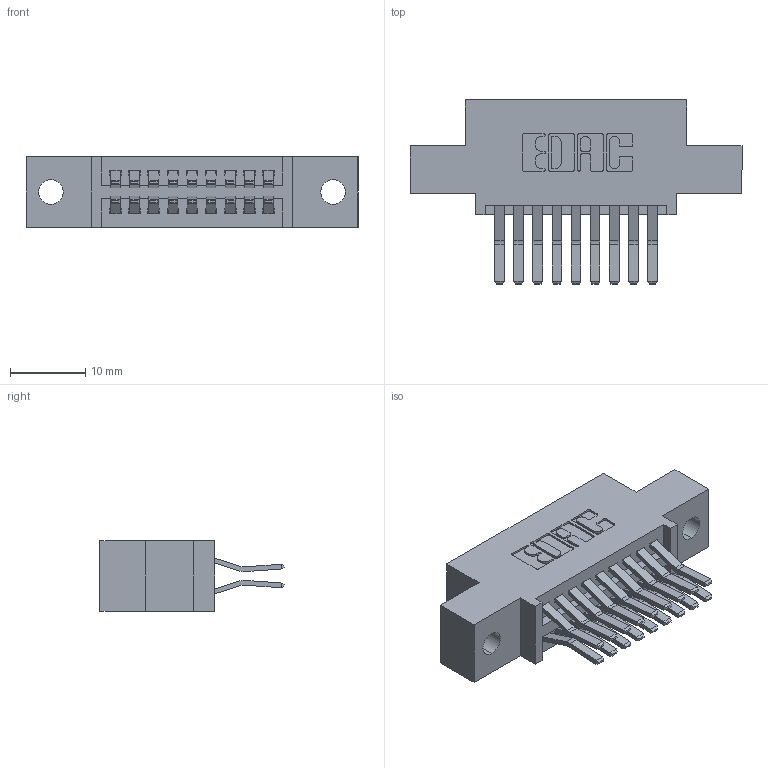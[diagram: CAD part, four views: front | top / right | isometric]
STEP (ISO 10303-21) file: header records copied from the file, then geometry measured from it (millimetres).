
FILE_DESCRIPTION (( 'STEP AP203' ), '1' );
FILE_NAME ('345-018-560-502.STEP', '2019-10-27T07:20:52', ( '' ), ( '' ), 'SwSTEP 2.0', 'SolidWorks 2016', '' );
FILE_SCHEMA (( 'CONFIG_CONTROL_DESIGN' ));
Length unit declared in the file: inch
Products named in the file (3): 345-292-001_560 Tail; 345 Part_0.110 Offset - 0.128 Dia; 345-018-560-502
Assembly tree (19 placements, depth 2):
  345-018-560-502
    345 Part_0.110 Offset - 0.128 Dia
    345-292-001_560 Tail  x18
Bounding box: 44.07 x 24.45 x 9.4 mm (x, y, z)
Volume: 3982.5 mm3; surface area: 5371.2 mm2
Topology: 19 solids, 19 shells, 1066 faces, 3143 edges, 2070 vertices
Faces by surface type: plane 678, cylinder 388
Entity records: 11727 total; most frequent: CARTESIAN_POINT 2000, ORIENTED_EDGE 1934, DIRECTION 1807, EDGE_CURVE 967, LINE 795, VECTOR 795, VERTEX_POINT 642, AXIS2_PLACEMENT_3D 506
